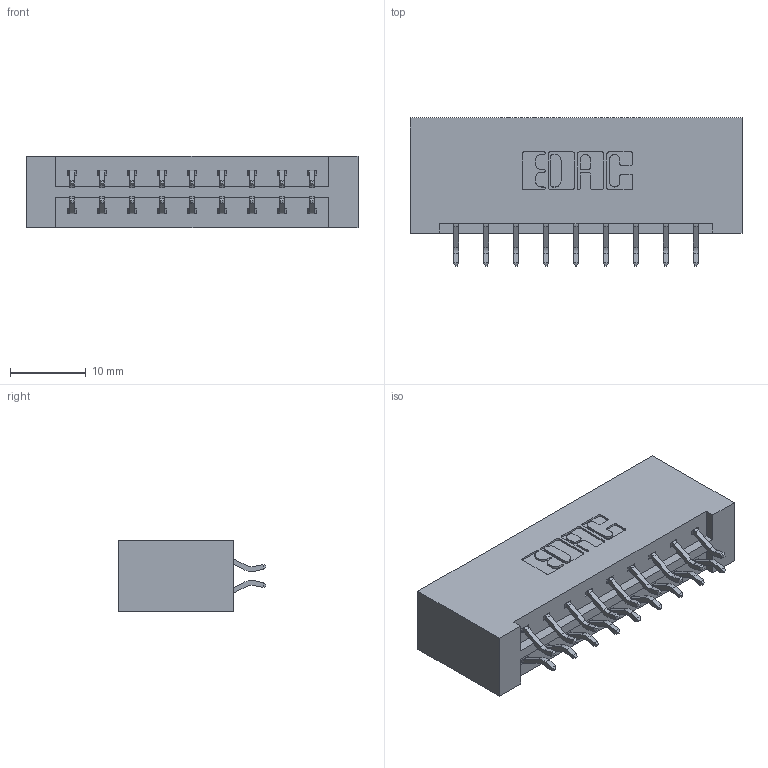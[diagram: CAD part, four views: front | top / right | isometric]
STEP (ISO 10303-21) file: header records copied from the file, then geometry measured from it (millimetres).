
FILE_DESCRIPTION (( 'STEP AP203' ), '1' );
FILE_NAME ('833-018-556-201.STEP', '2020-05-31T23:01:00', ( '' ), ( '' ), 'SwSTEP 2.0', 'SolidWorks 2020', '' );
FILE_SCHEMA (( 'CONFIG_CONTROL_DESIGN' ));
Length unit declared in the file: inch
Products named in the file (3): 833 Part_Lugless; 833-018-556-201; 345-292-001_556 Tail
Assembly tree (19 placements, depth 2):
  833-018-556-201
    833 Part_Lugless
    345-292-001_556 Tail  x18
Bounding box: 43.92 x 19.57 x 9.4 mm (x, y, z)
Volume: 4806.5 mm3; surface area: 5334.5 mm2
Topology: 19 solids, 19 shells, 1150 faces, 3401 edges, 2242 vertices
Faces by surface type: plane 786, cylinder 364
Entity records: 10001 total; most frequent: CARTESIAN_POINT 1710, ORIENTED_EDGE 1634, DIRECTION 1501, EDGE_CURVE 817, VECTOR 689, LINE 689, VERTEX_POINT 542, AXIS2_PLACEMENT_3D 406
